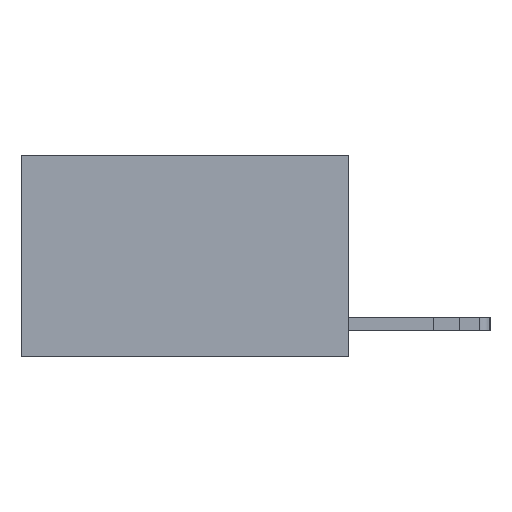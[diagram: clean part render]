
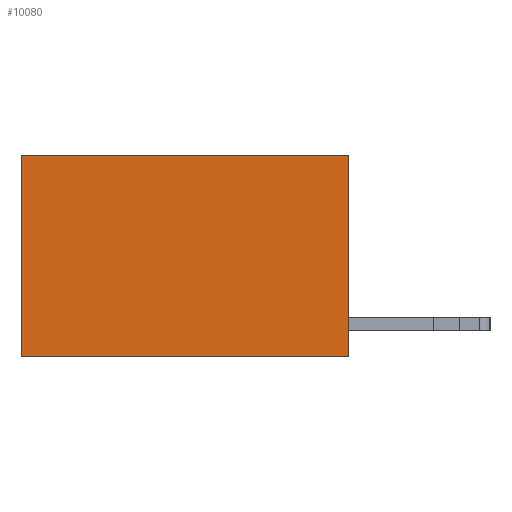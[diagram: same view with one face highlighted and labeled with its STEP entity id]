
A CAD part, left-side view. The second image highlights one B-rep face of the part: STEP entity #10080.
In plain terms, the highlighted planar face has unit normal (-1, 0, 0).
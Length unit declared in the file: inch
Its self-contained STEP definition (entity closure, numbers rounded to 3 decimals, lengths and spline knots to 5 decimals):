
#26 = VERTEX_POINT ( 'NONE', #10079 ) ;
#578 = VERTEX_POINT ( 'NONE', #9175 ) ;
#780 = LINE ( 'NONE', #6680, #2375 ) ;
#1514 = CARTESIAN_POINT ( 'NONE',  ( 0.2625, 0.6, 0. ) ) ;
#1863 = ORIENTED_EDGE ( 'NONE', *, *, #13491, .T. ) ;
#2375 = VECTOR ( 'NONE', #12459, 39.37008 ) ;
#2415 = VERTEX_POINT ( 'NONE', #17095 ) ;
#2726 = LINE ( 'NONE', #6801, #12079 ) ;
#3228 = DIRECTION ( 'NONE',  ( 0., 0., -1. ) ) ;
#3591 = PLANE ( 'NONE',  #14820 ) ;
#3786 = VECTOR ( 'NONE', #3228, 39.37008 ) ;
#4144 = CARTESIAN_POINT ( 'NONE',  ( 0.2625, 0., -0.37 ) ) ;
#4519 = EDGE_LOOP ( 'NONE', ( #12278, #9017, #13472, #1863 ) ) ;
#4595 = EDGE_CURVE ( 'NONE', #5593, #26, #780, .T. ) ;
#5466 = CARTESIAN_POINT ( 'NONE',  ( 0.2625, 0., 0. ) ) ;
#5593 = VERTEX_POINT ( 'NONE', #4144 ) ;
#6631 = FACE_OUTER_BOUND ( 'NONE', #4519, .T. ) ;
#6680 = CARTESIAN_POINT ( 'NONE',  ( 0.2625, 0., -0.37 ) ) ;
#6801 = CARTESIAN_POINT ( 'NONE',  ( 0.2625, 0., 0. ) ) ;
#7690 = CARTESIAN_POINT ( 'NONE',  ( 0.2625, 0., 0. ) ) ;
#9017 = ORIENTED_EDGE ( 'NONE', *, *, #4595, .F. ) ;
#9175 = CARTESIAN_POINT ( 'NONE',  ( 0.2625, 0.6, 0. ) ) ;
#9438 = DIRECTION ( 'NONE',  ( 1., 0., 0. ) ) ;
#9810 = EDGE_CURVE ( 'NONE', #578, #26, #17590, .T. ) ;
#9994 = DIRECTION ( 'NONE',  ( 0., 0., -1. ) ) ;
#10079 = CARTESIAN_POINT ( 'NONE',  ( 0.2625, 0.6, -0.37 ) ) ;
#10080 = ADVANCED_FACE ( 'NONE', ( #6631 ), #3591, .F. ) ;
#12079 = VECTOR ( 'NONE', #16008, 39.37008 ) ;
#12278 = ORIENTED_EDGE ( 'NONE', *, *, #9810, .T. ) ;
#12459 = DIRECTION ( 'NONE',  ( 0., 1., 0. ) ) ;
#13304 = VECTOR ( 'NONE', #9994, 39.37008 ) ;
#13472 = ORIENTED_EDGE ( 'NONE', *, *, #16425, .F. ) ;
#13491 = EDGE_CURVE ( 'NONE', #2415, #578, #2726, .T. ) ;
#13552 = DIRECTION ( 'NONE',  ( 0., 0., -1. ) ) ;
#14820 = AXIS2_PLACEMENT_3D ( 'NONE', #7690, #9438, #13552 ) ;
#16008 = DIRECTION ( 'NONE',  ( 0., 1., 0. ) ) ;
#16425 = EDGE_CURVE ( 'NONE', #2415, #5593, #18617, .T. ) ;
#17095 = CARTESIAN_POINT ( 'NONE',  ( 0.2625, 0., 0. ) ) ;
#17590 = LINE ( 'NONE', #1514, #3786 ) ;
#18617 = LINE ( 'NONE', #5466, #13304 ) ;
